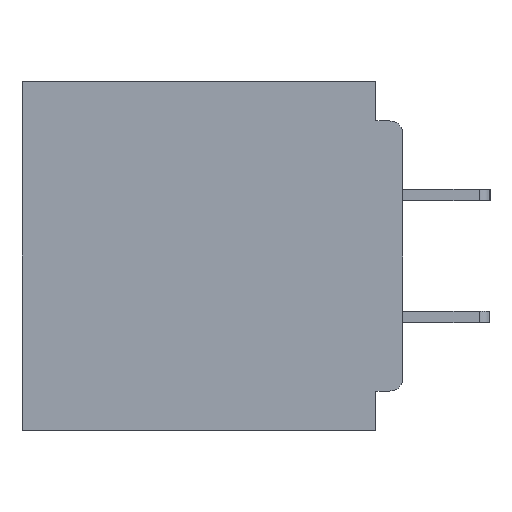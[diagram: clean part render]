
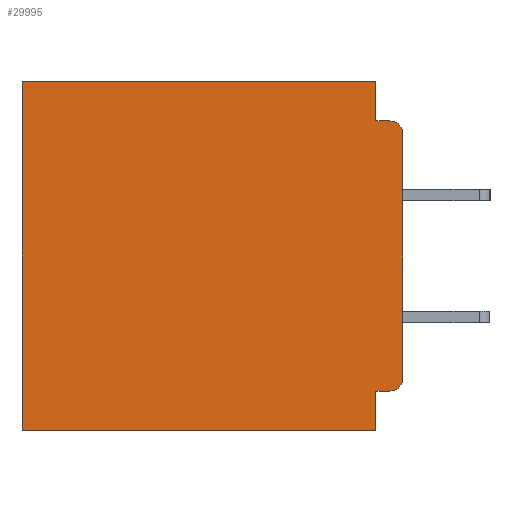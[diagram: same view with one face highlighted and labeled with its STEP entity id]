
A CAD part, left-side view. The second image highlights one B-rep face of the part: STEP entity #29995.
In plain terms, the highlighted planar face has unit normal (-1, 0, 0).
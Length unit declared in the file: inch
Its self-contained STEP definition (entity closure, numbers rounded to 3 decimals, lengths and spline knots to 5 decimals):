
#126 = LINE ( 'NONE', #13252, #26006 ) ;
#309 = VERTEX_POINT ( 'NONE', #11189 ) ;
#570 = ORIENTED_EDGE ( 'NONE', *, *, #7534, .F. ) ;
#1123 = CARTESIAN_POINT ( 'NONE',  ( 0.3, 0., -0.4 ) ) ;
#1875 = VERTEX_POINT ( 'NONE', #29148 ) ;
#2309 = VERTEX_POINT ( 'NONE', #4726 ) ;
#2830 = VECTOR ( 'NONE', #37101, 39.37008 ) ;
#3431 = CIRCLE ( 'NONE', #7173, 0.015 ) ;
#4085 = VERTEX_POINT ( 'NONE', #16180 ) ;
#4512 = FACE_OUTER_BOUND ( 'NONE', #44177, .T. ) ;
#4726 = CARTESIAN_POINT ( 'NONE',  ( 0.3, 0.031, 0. ) ) ;
#4963 = CARTESIAN_POINT ( 'NONE',  ( 0.3, 0.015, -0.34 ) ) ;
#5920 = VERTEX_POINT ( 'NONE', #14983 ) ;
#6526 = ORIENTED_EDGE ( 'NONE', *, *, #22998, .F. ) ;
#6593 = AXIS2_PLACEMENT_3D ( 'NONE', #4963, #29537, #8466 ) ;
#7173 = AXIS2_PLACEMENT_3D ( 'NONE', #16872, #41126, #20405 ) ;
#7333 = ORIENTED_EDGE ( 'NONE', *, *, #30034, .T. ) ;
#7534 = EDGE_CURVE ( 'NONE', #1875, #4085, #17129, .T. ) ;
#7767 = VERTEX_POINT ( 'NONE', #17577 ) ;
#8466 = DIRECTION ( 'NONE',  ( 0., 0., -1. ) ) ;
#8537 = VECTOR ( 'NONE', #13478, 39.37008 ) ;
#8888 = CARTESIAN_POINT ( 'NONE',  ( 0.3, 0.015, -0.355 ) ) ;
#8927 = AXIS2_PLACEMENT_3D ( 'NONE', #1123, #32697, #11738 ) ;
#9141 = CARTESIAN_POINT ( 'NONE',  ( 0.3, 0., -0.045 ) ) ;
#9401 = ORIENTED_EDGE ( 'NONE', *, *, #24744, .T. ) ;
#9938 = VERTEX_POINT ( 'NONE', #43179 ) ;
#10796 = ORIENTED_EDGE ( 'NONE', *, *, #16894, .F. ) ;
#11189 = CARTESIAN_POINT ( 'NONE',  ( 0.3, 0.015, -0.045 ) ) ;
#11385 = EDGE_CURVE ( 'NONE', #14122, #32819, #44483, .T. ) ;
#11565 = DIRECTION ( 'NONE',  ( 0., 0., -1. ) ) ;
#11738 = DIRECTION ( 'NONE',  ( 0., 0., -1. ) ) ;
#12196 = LINE ( 'NONE', #9141, #2830 ) ;
#12825 = CARTESIAN_POINT ( 'NONE',  ( 0.3, 0.031, 0. ) ) ;
#12829 = CARTESIAN_POINT ( 'NONE',  ( 0.3, 0., -0.4 ) ) ;
#13252 = CARTESIAN_POINT ( 'NONE',  ( 0.3, 0.031, -0.4 ) ) ;
#13478 = DIRECTION ( 'NONE',  ( 0., 1., 0. ) ) ;
#14122 = VERTEX_POINT ( 'NONE', #8888 ) ;
#14532 = LINE ( 'NONE', #16556, #32030 ) ;
#14983 = CARTESIAN_POINT ( 'NONE',  ( 0.3, 0.437, 0. ) ) ;
#16180 = CARTESIAN_POINT ( 'NONE',  ( 0.3, 0.437, -0.4 ) ) ;
#16217 = DIRECTION ( 'NONE',  ( 0., 1., 0. ) ) ;
#16556 = CARTESIAN_POINT ( 'NONE',  ( 0.3, 0.437, -0.4 ) ) ;
#16713 = DIRECTION ( 'NONE',  ( 0., 0., -1. ) ) ;
#16872 = CARTESIAN_POINT ( 'NONE',  ( 0.3, 0.015, -0.06 ) ) ;
#16894 = EDGE_CURVE ( 'NONE', #2309, #9938, #35017, .T. ) ;
#17129 = LINE ( 'NONE', #12829, #25363 ) ;
#17577 = CARTESIAN_POINT ( 'NONE',  ( 0.3, 0., -0.06 ) ) ;
#18580 = VECTOR ( 'NONE', #16217, 39.37008 ) ;
#20405 = DIRECTION ( 'NONE',  ( 0., 0., -1. ) ) ;
#20795 = EDGE_CURVE ( 'NONE', #7767, #309, #3431, .T. ) ;
#21786 = ORIENTED_EDGE ( 'NONE', *, *, #39971, .F. ) ;
#22998 = EDGE_CURVE ( 'NONE', #7767, #32997, #35076, .T. ) ;
#23249 = CIRCLE ( 'NONE', #6593, 0.015 ) ;
#23423 = DIRECTION ( 'NONE',  ( 0., 0., -1. ) ) ;
#24744 = EDGE_CURVE ( 'NONE', #2309, #5920, #28967, .T. ) ;
#25363 = VECTOR ( 'NONE', #26787, 39.37008 ) ;
#25605 = CARTESIAN_POINT ( 'NONE',  ( 0.3, 0., -0.34 ) ) ;
#25818 = VECTOR ( 'NONE', #23423, 39.37008 ) ;
#26006 = VECTOR ( 'NONE', #41042, 39.37008 ) ;
#26639 = CARTESIAN_POINT ( 'NONE',  ( 0.3, 0., 0. ) ) ;
#26787 = DIRECTION ( 'NONE',  ( 0., 1., 0. ) ) ;
#27702 = ORIENTED_EDGE ( 'NONE', *, *, #40511, .F. ) ;
#28967 = LINE ( 'NONE', #26639, #18580 ) ;
#29044 = CARTESIAN_POINT ( 'NONE',  ( 0.3, 0., -0.4 ) ) ;
#29148 = CARTESIAN_POINT ( 'NONE',  ( 0.3, 0.031, -0.4 ) ) ;
#29537 = DIRECTION ( 'NONE',  ( -1., 0., 0. ) ) ;
#29995 = ADVANCED_FACE ( 'NONE', ( #4512 ), #36017, .F. ) ;
#30034 = EDGE_CURVE ( 'NONE', #14122, #32997, #23249, .T. ) ;
#32030 = VECTOR ( 'NONE', #16713, 39.37008 ) ;
#32697 = DIRECTION ( 'NONE',  ( 1., 0., 0. ) ) ;
#32819 = VERTEX_POINT ( 'NONE', #35150 ) ;
#32997 = VERTEX_POINT ( 'NONE', #25605 ) ;
#35017 = LINE ( 'NONE', #12825, #25818 ) ;
#35076 = LINE ( 'NONE', #29044, #43099 ) ;
#35150 = CARTESIAN_POINT ( 'NONE',  ( 0.3, 0.031, -0.355 ) ) ;
#35301 = ORIENTED_EDGE ( 'NONE', *, *, #11385, .F. ) ;
#35332 = ORIENTED_EDGE ( 'NONE', *, *, #20795, .T. ) ;
#36017 = PLANE ( 'NONE',  #8927 ) ;
#36362 = EDGE_CURVE ( 'NONE', #5920, #4085, #14532, .T. ) ;
#37101 = DIRECTION ( 'NONE',  ( 0., -1., 0. ) ) ;
#37790 = ORIENTED_EDGE ( 'NONE', *, *, #36362, .T. ) ;
#37830 = CARTESIAN_POINT ( 'NONE',  ( 0.3, 0., -0.355 ) ) ;
#39971 = EDGE_CURVE ( 'NONE', #32819, #1875, #126, .T. ) ;
#40511 = EDGE_CURVE ( 'NONE', #9938, #309, #12196, .T. ) ;
#41042 = DIRECTION ( 'NONE',  ( 0., 0., -1. ) ) ;
#41126 = DIRECTION ( 'NONE',  ( -1., 0., 0. ) ) ;
#43099 = VECTOR ( 'NONE', #11565, 39.37008 ) ;
#43179 = CARTESIAN_POINT ( 'NONE',  ( 0.3, 0.031, -0.045 ) ) ;
#44177 = EDGE_LOOP ( 'NONE', ( #6526, #35332, #27702, #10796, #9401, #37790, #570, #21786, #35301, #7333 ) ) ;
#44483 = LINE ( 'NONE', #37830, #8537 ) ;
